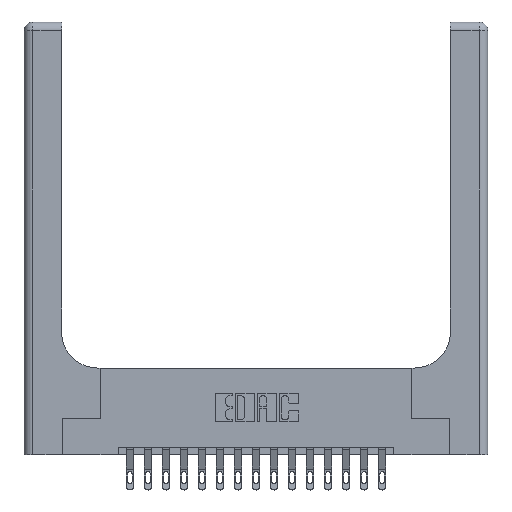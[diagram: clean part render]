
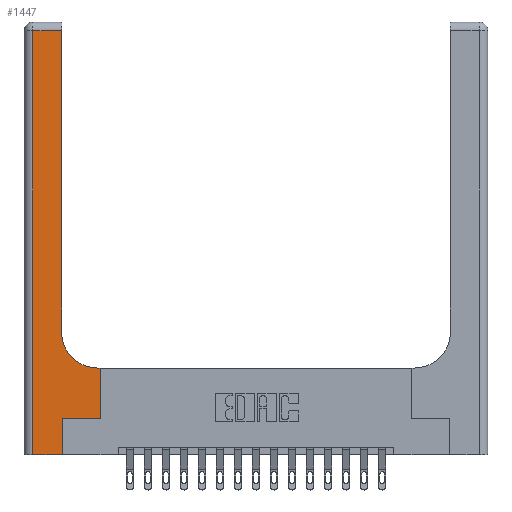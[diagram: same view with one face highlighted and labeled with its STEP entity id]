
A CAD part, top view. The second image highlights one B-rep face of the part: STEP entity #1447.
In plain terms, the highlighted planar face has unit normal (0, 0, 1).
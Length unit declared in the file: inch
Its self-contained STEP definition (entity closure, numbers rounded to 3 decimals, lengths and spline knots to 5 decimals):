
#50 = EDGE_CURVE ( 'NONE', #11909, #18000, #16869, .T. ) ;
#315 = LINE ( 'NONE', #10806, #8568 ) ;
#503 = LINE ( 'NONE', #18245, #9034 ) ;
#838 = CARTESIAN_POINT ( 'NONE',  ( 0.265, 0., 0.37 ) ) ;
#941 = ORIENTED_EDGE ( 'NONE', *, *, #10616, .T. ) ;
#977 = CARTESIAN_POINT ( 'NONE',  ( 0.26, 2.94, 0.37 ) ) ;
#1088 = AXIS2_PLACEMENT_3D ( 'NONE', #5615, #11617, #17576 ) ;
#1108 = PLANE ( 'NONE',  #1088 ) ;
#1132 = ORIENTED_EDGE ( 'NONE', *, *, #11323, .T. ) ;
#1435 = VECTOR ( 'NONE', #2923, 39.37008 ) ;
#1447 = ADVANCED_FACE ( 'NONE', ( #12789 ), #1108, .F. ) ;
#1492 = VECTOR ( 'NONE', #8715, 39.37008 ) ;
#1502 = CARTESIAN_POINT ( 'NONE',  ( 0.51, 0.85, 0.37 ) ) ;
#1684 = CARTESIAN_POINT ( 'NONE',  ( 0.26, 3., 0.37 ) ) ;
#1723 = DIRECTION ( 'NONE',  ( 0., 1., 0. ) ) ;
#1835 = CARTESIAN_POINT ( 'NONE',  ( 0.26, 0.85, 0.37 ) ) ;
#2210 = CIRCLE ( 'NONE', #18508, 0.25 ) ;
#2386 = VERTEX_POINT ( 'NONE', #2824 ) ;
#2443 = VERTEX_POINT ( 'NONE', #17533 ) ;
#2537 = EDGE_LOOP ( 'NONE', ( #4380, #17148, #18775, #13137, #941, #1132, #11863, #12279, #2782 ) ) ;
#2782 = ORIENTED_EDGE ( 'NONE', *, *, #12828, .T. ) ;
#2824 = CARTESIAN_POINT ( 'NONE',  ( 0.528, 0.6, 0.37 ) ) ;
#2923 = DIRECTION ( 'NONE',  ( 1., 0., 0. ) ) ;
#3641 = EDGE_CURVE ( 'NONE', #4173, #13424, #5759, .T. ) ;
#4173 = VERTEX_POINT ( 'NONE', #18201 ) ;
#4303 = CARTESIAN_POINT ( 'NONE',  ( 0.51, 0.6, 0.37 ) ) ;
#4380 = ORIENTED_EDGE ( 'NONE', *, *, #50, .T. ) ;
#4478 = CARTESIAN_POINT ( 'NONE',  ( 0.265, 0.25, 0.37 ) ) ;
#4552 = LINE ( 'NONE', #13878, #13910 ) ;
#4786 = DIRECTION ( 'NONE',  ( -1., 0., 0. ) ) ;
#4997 = CARTESIAN_POINT ( 'NONE',  ( 0.528, 0.25, 0.37 ) ) ;
#5615 = CARTESIAN_POINT ( 'NONE',  ( 0., 3., 0.37 ) ) ;
#5759 = LINE ( 'NONE', #14696, #1435 ) ;
#6274 = DIRECTION ( 'NONE',  ( 0., -1., 0. ) ) ;
#7671 = DIRECTION ( 'NONE',  ( 0., 1., 0. ) ) ;
#7796 = DIRECTION ( 'NONE',  ( 1., 0., 0. ) ) ;
#8227 = EDGE_CURVE ( 'NONE', #2386, #15756, #503, .T. ) ;
#8327 = CARTESIAN_POINT ( 'NONE',  ( 0.265, 0., 0.37 ) ) ;
#8568 = VECTOR ( 'NONE', #6274, 39.37008 ) ;
#8715 = DIRECTION ( 'NONE',  ( 0., 1., 0. ) ) ;
#9034 = VECTOR ( 'NONE', #4786, 39.37008 ) ;
#10002 = LINE ( 'NONE', #8327, #1492 ) ;
#10616 = EDGE_CURVE ( 'NONE', #13424, #15238, #10002, .T. ) ;
#10758 = VECTOR ( 'NONE', #16499, 39.37008 ) ;
#10806 = CARTESIAN_POINT ( 'NONE',  ( 0.06, 3., 0.37 ) ) ;
#11323 = EDGE_CURVE ( 'NONE', #15238, #15561, #16887, .T. ) ;
#11617 = DIRECTION ( 'NONE',  ( 0., 0., -1. ) ) ;
#11863 = ORIENTED_EDGE ( 'NONE', *, *, #18740, .T. ) ;
#11909 = VERTEX_POINT ( 'NONE', #1835 ) ;
#12279 = ORIENTED_EDGE ( 'NONE', *, *, #8227, .T. ) ;
#12789 = FACE_OUTER_BOUND ( 'NONE', #2537, .T. ) ;
#12828 = EDGE_CURVE ( 'NONE', #15756, #11909, #2210, .T. ) ;
#13137 = ORIENTED_EDGE ( 'NONE', *, *, #3641, .T. ) ;
#13424 = VERTEX_POINT ( 'NONE', #838 ) ;
#13461 = DIRECTION ( 'NONE',  ( 1., 0., 0. ) ) ;
#13470 = LINE ( 'NONE', #16030, #10758 ) ;
#13878 = CARTESIAN_POINT ( 'NONE',  ( 0.528, 0.25, 0.37 ) ) ;
#13910 = VECTOR ( 'NONE', #1723, 39.37008 ) ;
#13960 = CARTESIAN_POINT ( 'NONE',  ( 0.265, 0.25, 0.37 ) ) ;
#14010 = VECTOR ( 'NONE', #7796, 39.37008 ) ;
#14421 = VECTOR ( 'NONE', #7671, 39.37008 ) ;
#14696 = CARTESIAN_POINT ( 'NONE',  ( 0., 0., 0.37 ) ) ;
#15238 = VERTEX_POINT ( 'NONE', #4478 ) ;
#15561 = VERTEX_POINT ( 'NONE', #4997 ) ;
#15756 = VERTEX_POINT ( 'NONE', #4303 ) ;
#16030 = CARTESIAN_POINT ( 'NONE',  ( 0., 2.94, 0.37 ) ) ;
#16499 = DIRECTION ( 'NONE',  ( -1., 0., 0. ) ) ;
#16869 = LINE ( 'NONE', #1684, #14421 ) ;
#16887 = LINE ( 'NONE', #13960, #14010 ) ;
#17148 = ORIENTED_EDGE ( 'NONE', *, *, #17475, .T. ) ;
#17475 = EDGE_CURVE ( 'NONE', #18000, #2443, #13470, .T. ) ;
#17533 = CARTESIAN_POINT ( 'NONE',  ( 0.06, 2.94, 0.37 ) ) ;
#17576 = DIRECTION ( 'NONE',  ( -1., 0., 0. ) ) ;
#17671 = DIRECTION ( 'NONE',  ( 0., 0., -1. ) ) ;
#17877 = EDGE_CURVE ( 'NONE', #2443, #4173, #315, .T. ) ;
#18000 = VERTEX_POINT ( 'NONE', #977 ) ;
#18201 = CARTESIAN_POINT ( 'NONE',  ( 0.06, 0., 0.37 ) ) ;
#18245 = CARTESIAN_POINT ( 'NONE',  ( 0.26, 0.6, 0.37 ) ) ;
#18508 = AXIS2_PLACEMENT_3D ( 'NONE', #1502, #17671, #13461 ) ;
#18740 = EDGE_CURVE ( 'NONE', #15561, #2386, #4552, .T. ) ;
#18775 = ORIENTED_EDGE ( 'NONE', *, *, #17877, .T. ) ;
